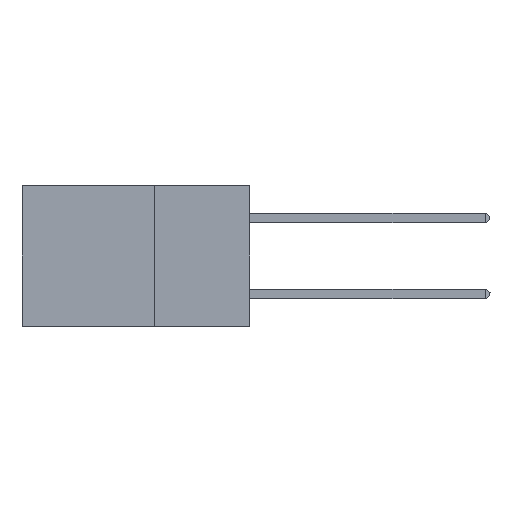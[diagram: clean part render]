
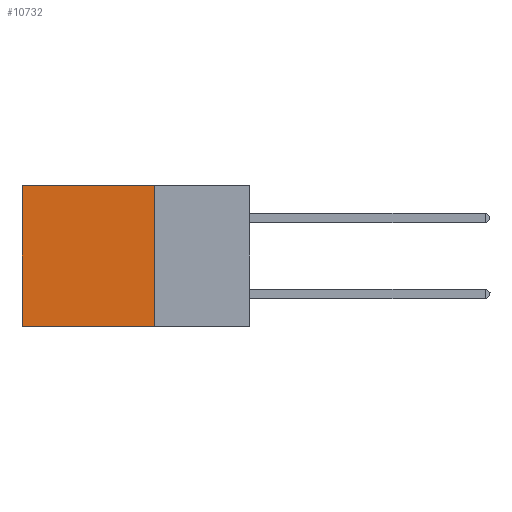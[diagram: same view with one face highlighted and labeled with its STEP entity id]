
A CAD part, left-side view. The second image highlights one B-rep face of the part: STEP entity #10732.
In plain terms, the highlighted planar face has unit normal (-1, 0, 0).
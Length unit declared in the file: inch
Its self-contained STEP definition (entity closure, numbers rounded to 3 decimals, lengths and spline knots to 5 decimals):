
#945 = LINE ( 'NONE', #24943, #23172 ) ;
#1259 = VECTOR ( 'NONE', #20197, 39.37008 ) ;
#1313 = EDGE_LOOP ( 'NONE', ( #22925, #2300, #28424, #2667 ) ) ;
#1414 = PLANE ( 'NONE',  #1664 ) ;
#1487 = CARTESIAN_POINT ( 'NONE',  ( 0.2875, 0.25, 0. ) ) ;
#1664 = AXIS2_PLACEMENT_3D ( 'NONE', #24358, #5894, #28519 ) ;
#2082 = VERTEX_POINT ( 'NONE', #2622 ) ;
#2300 = ORIENTED_EDGE ( 'NONE', *, *, #16761, .F. ) ;
#2622 = CARTESIAN_POINT ( 'NONE',  ( 0.2875, 0.6, -0.37 ) ) ;
#2667 = ORIENTED_EDGE ( 'NONE', *, *, #23839, .T. ) ;
#3022 = LINE ( 'NONE', #6207, #1259 ) ;
#3386 = DIRECTION ( 'NONE',  ( 0., 1., 0. ) ) ;
#5884 = CARTESIAN_POINT ( 'NONE',  ( 0.2875, 0.25, -0.37 ) ) ;
#5894 = DIRECTION ( 'NONE',  ( 1., 0., 0. ) ) ;
#6207 = CARTESIAN_POINT ( 'NONE',  ( 0.2875, 0.6, 0. ) ) ;
#6326 = DIRECTION ( 'NONE',  ( 0., 1., 0. ) ) ;
#9325 = EDGE_CURVE ( 'NONE', #27570, #22612, #945, .T. ) ;
#10732 = ADVANCED_FACE ( 'NONE', ( #12991 ), #1414, .F. ) ;
#12059 = LINE ( 'NONE', #5884, #29624 ) ;
#12991 = FACE_OUTER_BOUND ( 'NONE', #1313, .T. ) ;
#16761 = EDGE_CURVE ( 'NONE', #22612, #2082, #12059, .T. ) ;
#18058 = EDGE_CURVE ( 'NONE', #20027, #2082, #3022, .T. ) ;
#18061 = CARTESIAN_POINT ( 'NONE',  ( 0.2875, 0.25, -0.37 ) ) ;
#18092 = CARTESIAN_POINT ( 'NONE',  ( 0.2875, 0.25, 0. ) ) ;
#20027 = VERTEX_POINT ( 'NONE', #26514 ) ;
#20197 = DIRECTION ( 'NONE',  ( 0., 0., -1. ) ) ;
#22612 = VERTEX_POINT ( 'NONE', #18061 ) ;
#22925 = ORIENTED_EDGE ( 'NONE', *, *, #18058, .T. ) ;
#22975 = VECTOR ( 'NONE', #6326, 39.37008 ) ;
#23172 = VECTOR ( 'NONE', #29516, 39.37008 ) ;
#23839 = EDGE_CURVE ( 'NONE', #27570, #20027, #29002, .T. ) ;
#24358 = CARTESIAN_POINT ( 'NONE',  ( 0.2875, 0.25, 0. ) ) ;
#24943 = CARTESIAN_POINT ( 'NONE',  ( 0.2875, 0.25, 0. ) ) ;
#26514 = CARTESIAN_POINT ( 'NONE',  ( 0.2875, 0.6, 0. ) ) ;
#27570 = VERTEX_POINT ( 'NONE', #1487 ) ;
#28424 = ORIENTED_EDGE ( 'NONE', *, *, #9325, .F. ) ;
#28519 = DIRECTION ( 'NONE',  ( 0., 0., -1. ) ) ;
#29002 = LINE ( 'NONE', #18092, #22975 ) ;
#29516 = DIRECTION ( 'NONE',  ( 0., 0., -1. ) ) ;
#29624 = VECTOR ( 'NONE', #3386, 39.37008 ) ;
